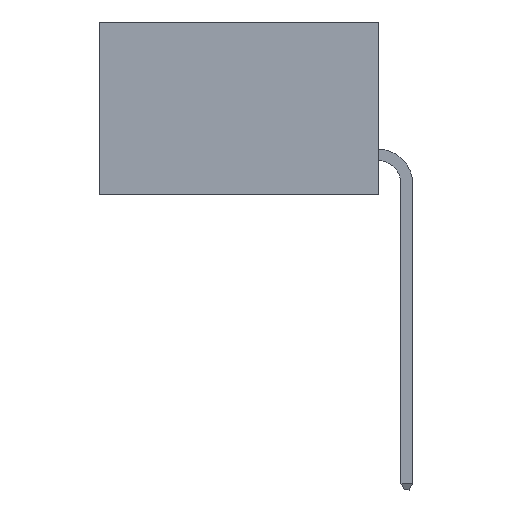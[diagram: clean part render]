
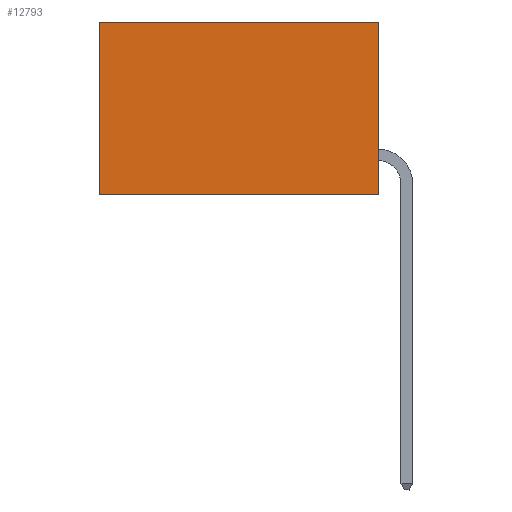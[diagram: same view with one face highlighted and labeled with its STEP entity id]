
A CAD part, left-side view. The second image highlights one B-rep face of the part: STEP entity #12793.
In plain terms, the highlighted planar face has unit normal (-1, 0, 0).
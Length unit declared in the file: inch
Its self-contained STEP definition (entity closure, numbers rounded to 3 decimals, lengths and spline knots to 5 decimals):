
#461 = ORIENTED_EDGE ( 'NONE', *, *, #16544, .T. ) ;
#1157 = EDGE_CURVE ( 'NONE', #16169, #11350, #14908, .T. ) ;
#1197 = CARTESIAN_POINT ( 'NONE',  ( 0.298, 0., 0. ) ) ;
#1529 = ORIENTED_EDGE ( 'NONE', *, *, #14643, .T. ) ;
#2996 = CARTESIAN_POINT ( 'NONE',  ( 0.298, 0.6, -0.37 ) ) ;
#3331 = DIRECTION ( 'NONE',  ( 0., 1., 0. ) ) ;
#3525 = VERTEX_POINT ( 'NONE', #1197 ) ;
#4582 = VECTOR ( 'NONE', #5973, 39.37008 ) ;
#4768 = VERTEX_POINT ( 'NONE', #16014 ) ;
#5973 = DIRECTION ( 'NONE',  ( 0., 0., -1. ) ) ;
#7853 = LINE ( 'NONE', #13786, #4582 ) ;
#7891 = EDGE_CURVE ( 'NONE', #3525, #16169, #7853, .T. ) ;
#8107 = FACE_OUTER_BOUND ( 'NONE', #12062, .T. ) ;
#8368 = ORIENTED_EDGE ( 'NONE', *, *, #7891, .F. ) ;
#8468 = DIRECTION ( 'NONE',  ( 0., 0., -1. ) ) ;
#8983 = CARTESIAN_POINT ( 'NONE',  ( 0.298, 0.6, 0. ) ) ;
#9185 = AXIS2_PLACEMENT_3D ( 'NONE', #16215, #16271, #8468 ) ;
#9847 = DIRECTION ( 'NONE',  ( 0., 1., 0. ) ) ;
#10385 = VECTOR ( 'NONE', #3331, 39.37008 ) ;
#11286 = VECTOR ( 'NONE', #13029, 39.37008 ) ;
#11350 = VERTEX_POINT ( 'NONE', #2996 ) ;
#12048 = CARTESIAN_POINT ( 'NONE',  ( 0.298, 0., -0.37 ) ) ;
#12062 = EDGE_LOOP ( 'NONE', ( #1529, #13799, #8368, #461 ) ) ;
#12793 = ADVANCED_FACE ( 'NONE', ( #8107 ), #13660, .F. ) ;
#13029 = DIRECTION ( 'NONE',  ( 0., 0., -1. ) ) ;
#13496 = CARTESIAN_POINT ( 'NONE',  ( 0.298, 0., 0. ) ) ;
#13660 = PLANE ( 'NONE',  #9185 ) ;
#13786 = CARTESIAN_POINT ( 'NONE',  ( 0.298, 0., 0. ) ) ;
#13799 = ORIENTED_EDGE ( 'NONE', *, *, #1157, .F. ) ;
#14643 = EDGE_CURVE ( 'NONE', #4768, #11350, #15773, .T. ) ;
#14908 = LINE ( 'NONE', #12048, #16325 ) ;
#15584 = CARTESIAN_POINT ( 'NONE',  ( 0.298, 0., -0.37 ) ) ;
#15773 = LINE ( 'NONE', #8983, #11286 ) ;
#15902 = LINE ( 'NONE', #13496, #10385 ) ;
#16014 = CARTESIAN_POINT ( 'NONE',  ( 0.298, 0.6, 0. ) ) ;
#16169 = VERTEX_POINT ( 'NONE', #15584 ) ;
#16215 = CARTESIAN_POINT ( 'NONE',  ( 0.298, 0., 0. ) ) ;
#16271 = DIRECTION ( 'NONE',  ( 1., 0., 0. ) ) ;
#16325 = VECTOR ( 'NONE', #9847, 39.37008 ) ;
#16544 = EDGE_CURVE ( 'NONE', #3525, #4768, #15902, .T. ) ;
